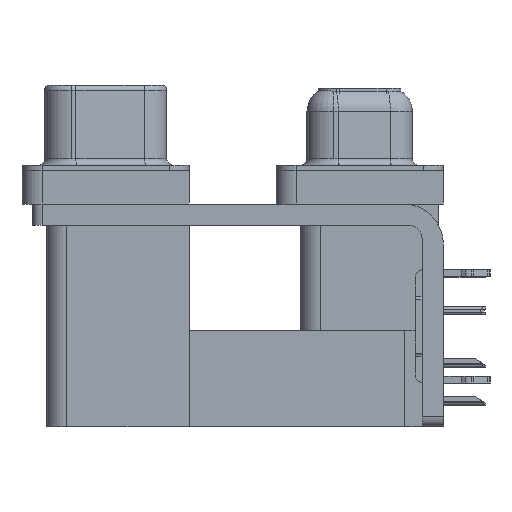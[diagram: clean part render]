
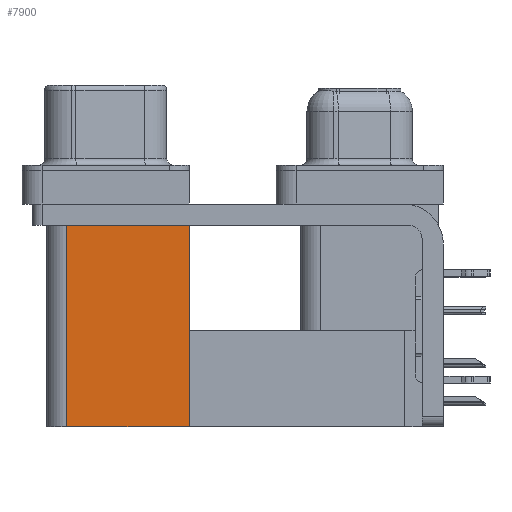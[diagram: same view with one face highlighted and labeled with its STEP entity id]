
A CAD part, left-side view. The second image highlights one B-rep face of the part: STEP entity #7900.
In plain terms, the highlighted planar face has unit normal (-1, 0, 0).
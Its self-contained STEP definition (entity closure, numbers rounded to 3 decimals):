
#957 = AXIS2_PLACEMENT_3D ( 'NONE', #33708, #47395, #33998 ) ;
#1042 = DIRECTION ( 'NONE',  ( 0., 0., 1. ) ) ;
#4813 = CARTESIAN_POINT ( 'NONE',  ( 3.7, 12.775, -2.5 ) ) ;
#4956 = EDGE_CURVE ( 'NONE', #13031, #15055, #25691, .T. ) ;
#5766 = LINE ( 'NONE', #18337, #42609 ) ;
#6944 = VERTEX_POINT ( 'NONE', #16129 ) ;
#7900 = ADVANCED_FACE ( 'NONE', ( #26467 ), #46557, .F. ) ;
#11948 = EDGE_CURVE ( 'NONE', #6944, #13097, #5766, .T. ) ;
#13002 = VECTOR ( 'NONE', #21810, 1000. ) ;
#13031 = VERTEX_POINT ( 'NONE', #28901 ) ;
#13097 = VERTEX_POINT ( 'NONE', #41729 ) ;
#15055 = VERTEX_POINT ( 'NONE', #19357 ) ;
#15634 = CARTESIAN_POINT ( 'NONE',  ( 3.7, 12.775, -19.2 ) ) ;
#16129 = CARTESIAN_POINT ( 'NONE',  ( 3.7, 12.775, -19.2 ) ) ;
#16209 = ORIENTED_EDGE ( 'NONE', *, *, #24504, .F. ) ;
#17630 = DIRECTION ( 'NONE',  ( 0., 0., 1. ) ) ;
#18337 = CARTESIAN_POINT ( 'NONE',  ( 3.7, 12.775, -19.2 ) ) ;
#19160 = ORIENTED_EDGE ( 'NONE', *, *, #11948, .T. ) ;
#19357 = CARTESIAN_POINT ( 'NONE',  ( 3.7, 21.975, -2.5 ) ) ;
#20208 = ORIENTED_EDGE ( 'NONE', *, *, #4956, .F. ) ;
#21810 = DIRECTION ( 'NONE',  ( 0., 1., 0. ) ) ;
#22078 = LINE ( 'NONE', #4813, #13002 ) ;
#24504 = EDGE_CURVE ( 'NONE', #6944, #13031, #49889, .T. ) ;
#25691 = LINE ( 'NONE', #47159, #39260 ) ;
#26159 = EDGE_CURVE ( 'NONE', #13097, #15055, #22078, .T. ) ;
#26467 = FACE_OUTER_BOUND ( 'NONE', #48311, .T. ) ;
#28901 = CARTESIAN_POINT ( 'NONE',  ( 3.7, 21.975, -19.2 ) ) ;
#33708 = CARTESIAN_POINT ( 'NONE',  ( 3.7, 12.775, -19.2 ) ) ;
#33998 = DIRECTION ( 'NONE',  ( 0., 1., 0. ) ) ;
#36785 = DIRECTION ( 'NONE',  ( 0., 1., 0. ) ) ;
#38776 = VECTOR ( 'NONE', #36785, 1000. ) ;
#39260 = VECTOR ( 'NONE', #17630, 1000. ) ;
#41729 = CARTESIAN_POINT ( 'NONE',  ( 3.7, 12.775, -2.5 ) ) ;
#42609 = VECTOR ( 'NONE', #1042, 1000. ) ;
#46557 = PLANE ( 'NONE',  #957 ) ;
#47159 = CARTESIAN_POINT ( 'NONE',  ( 3.7, 21.975, -19.2 ) ) ;
#47395 = DIRECTION ( 'NONE',  ( 1., 0., 0. ) ) ;
#48311 = EDGE_LOOP ( 'NONE', ( #54964, #20208, #16209, #19160 ) ) ;
#49889 = LINE ( 'NONE', #15634, #38776 ) ;
#54964 = ORIENTED_EDGE ( 'NONE', *, *, #26159, .T. ) ;
